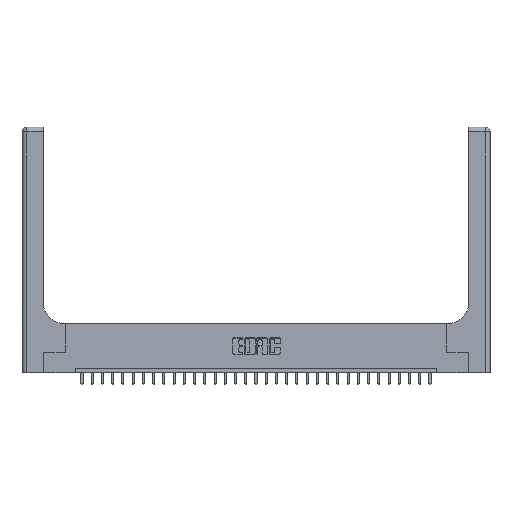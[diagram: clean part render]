
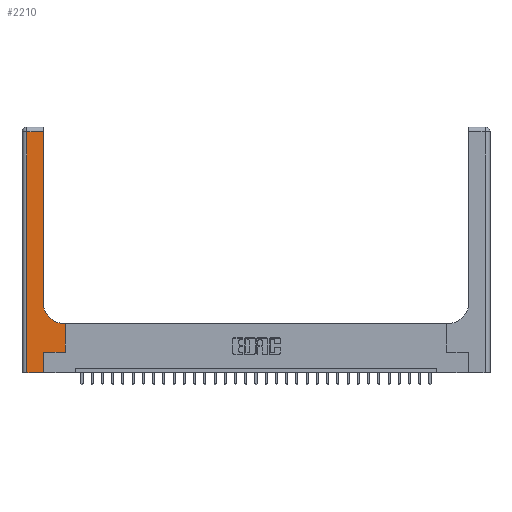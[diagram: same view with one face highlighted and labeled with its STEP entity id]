
A CAD part, top view. The second image highlights one B-rep face of the part: STEP entity #2210.
In plain terms, the highlighted planar face has unit normal (0, 0, 1).
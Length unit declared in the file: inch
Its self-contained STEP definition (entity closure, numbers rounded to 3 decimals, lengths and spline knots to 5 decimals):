
#123 = DIRECTION ( 'NONE',  ( 0., -1., 0. ) ) ;
#507 = VECTOR ( 'NONE', #12586, 39.37008 ) ;
#1321 = ORIENTED_EDGE ( 'NONE', *, *, #25580, .T. ) ;
#1809 = LINE ( 'NONE', #22933, #21004 ) ;
#2071 = VERTEX_POINT ( 'NONE', #10616 ) ;
#2144 = VERTEX_POINT ( 'NONE', #11630 ) ;
#2210 = ADVANCED_FACE ( 'NONE', ( #9789 ), #18797, .F. ) ;
#2477 = CIRCLE ( 'NONE', #15744, 0.25 ) ;
#3030 = ORIENTED_EDGE ( 'NONE', *, *, #11332, .T. ) ;
#3154 = ORIENTED_EDGE ( 'NONE', *, *, #12358, .T. ) ;
#3342 = EDGE_CURVE ( 'NONE', #7625, #2071, #5668, .T. ) ;
#3487 = CARTESIAN_POINT ( 'NONE',  ( 0.26, 0.6, 0.37 ) ) ;
#4273 = CARTESIAN_POINT ( 'NONE',  ( 0.265, 0., 0.37 ) ) ;
#4502 = LINE ( 'NONE', #19215, #507 ) ;
#4661 = DIRECTION ( 'NONE',  ( -1., 0., 0. ) ) ;
#4946 = LINE ( 'NONE', #17472, #9366 ) ;
#5002 = LINE ( 'NONE', #24192, #11797 ) ;
#5167 = CARTESIAN_POINT ( 'NONE',  ( 0.26, 3., 0.37 ) ) ;
#5451 = DIRECTION ( 'NONE',  ( 0., 0., -1. ) ) ;
#5549 = ORIENTED_EDGE ( 'NONE', *, *, #3342, .T. ) ;
#5668 = LINE ( 'NONE', #5938, #27555 ) ;
#5938 = CARTESIAN_POINT ( 'NONE',  ( 0.528, 0.25, 0.37 ) ) ;
#6461 = VERTEX_POINT ( 'NONE', #24330 ) ;
#7625 = VERTEX_POINT ( 'NONE', #25253 ) ;
#8441 = CARTESIAN_POINT ( 'NONE',  ( 0.06, 0., 0.37 ) ) ;
#8455 = EDGE_CURVE ( 'NONE', #19515, #6461, #17638, .T. ) ;
#9366 = VECTOR ( 'NONE', #4661, 39.37008 ) ;
#9689 = DIRECTION ( 'NONE',  ( 1., 0., 0. ) ) ;
#9789 = FACE_OUTER_BOUND ( 'NONE', #10836, .T. ) ;
#10319 = ORIENTED_EDGE ( 'NONE', *, *, #8455, .T. ) ;
#10358 = CARTESIAN_POINT ( 'NONE',  ( 0.26, 0.85, 0.37 ) ) ;
#10376 = CARTESIAN_POINT ( 'NONE',  ( 0., 3., 0.37 ) ) ;
#10616 = CARTESIAN_POINT ( 'NONE',  ( 0.528, 0.6, 0.37 ) ) ;
#10676 = AXIS2_PLACEMENT_3D ( 'NONE', #10376, #5451, #16843 ) ;
#10683 = VERTEX_POINT ( 'NONE', #24503 ) ;
#10836 = EDGE_LOOP ( 'NONE', ( #10319, #18321, #3030, #3154, #24877, #27242, #5549, #1321, #23144 ) ) ;
#11332 = EDGE_CURVE ( 'NONE', #2144, #21987, #5002, .T. ) ;
#11630 = CARTESIAN_POINT ( 'NONE',  ( 0.06, 2.94, 0.37 ) ) ;
#11797 = VECTOR ( 'NONE', #123, 39.37008 ) ;
#12358 = EDGE_CURVE ( 'NONE', #21987, #27604, #14657, .T. ) ;
#12586 = DIRECTION ( 'NONE',  ( 0., 1., 0. ) ) ;
#13302 = EDGE_CURVE ( 'NONE', #14321, #7625, #1809, .T. ) ;
#14111 = DIRECTION ( 'NONE',  ( 1., 0., 0. ) ) ;
#14321 = VERTEX_POINT ( 'NONE', #24060 ) ;
#14356 = DIRECTION ( 'NONE',  ( -1., 0., 0. ) ) ;
#14657 = LINE ( 'NONE', #22748, #15994 ) ;
#15744 = AXIS2_PLACEMENT_3D ( 'NONE', #20662, #16327, #14111 ) ;
#15994 = VECTOR ( 'NONE', #9689, 39.37008 ) ;
#16327 = DIRECTION ( 'NONE',  ( 0., 0., -1. ) ) ;
#16713 = EDGE_CURVE ( 'NONE', #6461, #2144, #4946, .T. ) ;
#16744 = DIRECTION ( 'NONE',  ( 0., 1., 0. ) ) ;
#16843 = DIRECTION ( 'NONE',  ( -1., 0., 0. ) ) ;
#17472 = CARTESIAN_POINT ( 'NONE',  ( 0., 2.94, 0.37 ) ) ;
#17638 = LINE ( 'NONE', #5167, #18983 ) ;
#17955 = VECTOR ( 'NONE', #14356, 39.37008 ) ;
#18297 = LINE ( 'NONE', #3487, #17955 ) ;
#18321 = ORIENTED_EDGE ( 'NONE', *, *, #16713, .T. ) ;
#18797 = PLANE ( 'NONE',  #10676 ) ;
#18983 = VECTOR ( 'NONE', #16744, 39.37008 ) ;
#19106 = DIRECTION ( 'NONE',  ( 0., 1., 0. ) ) ;
#19215 = CARTESIAN_POINT ( 'NONE',  ( 0.265, 0., 0.37 ) ) ;
#19515 = VERTEX_POINT ( 'NONE', #10358 ) ;
#20132 = EDGE_CURVE ( 'NONE', #27604, #14321, #4502, .T. ) ;
#20578 = DIRECTION ( 'NONE',  ( 1., 0., 0. ) ) ;
#20662 = CARTESIAN_POINT ( 'NONE',  ( 0.51, 0.85, 0.37 ) ) ;
#20895 = EDGE_CURVE ( 'NONE', #10683, #19515, #2477, .T. ) ;
#21004 = VECTOR ( 'NONE', #20578, 39.37008 ) ;
#21987 = VERTEX_POINT ( 'NONE', #8441 ) ;
#22748 = CARTESIAN_POINT ( 'NONE',  ( 0., 0., 0.37 ) ) ;
#22933 = CARTESIAN_POINT ( 'NONE',  ( 0.265, 0.25, 0.37 ) ) ;
#23144 = ORIENTED_EDGE ( 'NONE', *, *, #20895, .T. ) ;
#24060 = CARTESIAN_POINT ( 'NONE',  ( 0.265, 0.25, 0.37 ) ) ;
#24192 = CARTESIAN_POINT ( 'NONE',  ( 0.06, 3., 0.37 ) ) ;
#24330 = CARTESIAN_POINT ( 'NONE',  ( 0.26, 2.94, 0.37 ) ) ;
#24503 = CARTESIAN_POINT ( 'NONE',  ( 0.51, 0.6, 0.37 ) ) ;
#24877 = ORIENTED_EDGE ( 'NONE', *, *, #20132, .T. ) ;
#25253 = CARTESIAN_POINT ( 'NONE',  ( 0.528, 0.25, 0.37 ) ) ;
#25580 = EDGE_CURVE ( 'NONE', #2071, #10683, #18297, .T. ) ;
#27242 = ORIENTED_EDGE ( 'NONE', *, *, #13302, .T. ) ;
#27555 = VECTOR ( 'NONE', #19106, 39.37008 ) ;
#27604 = VERTEX_POINT ( 'NONE', #4273 ) ;
